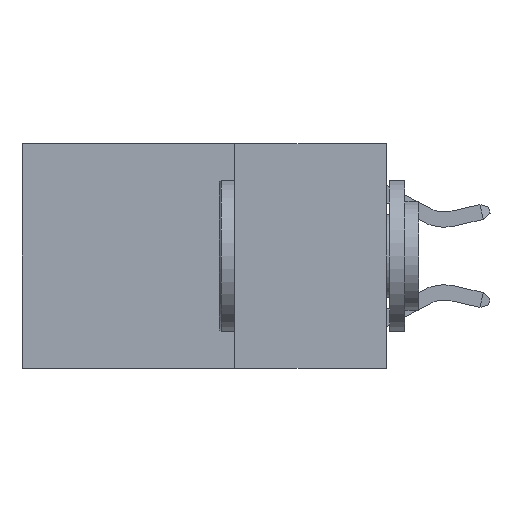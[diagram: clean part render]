
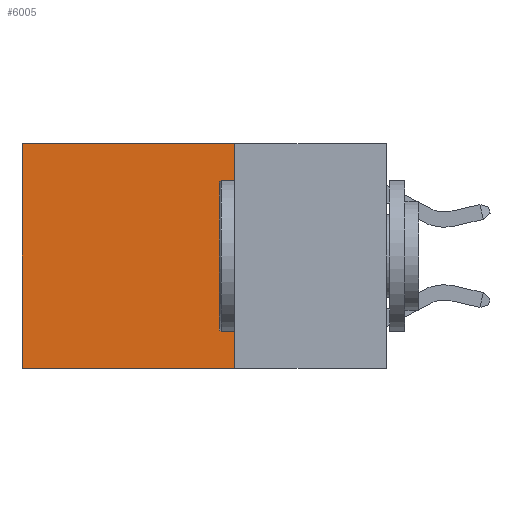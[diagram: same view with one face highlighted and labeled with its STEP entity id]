
A CAD part, left-side view. The second image highlights one B-rep face of the part: STEP entity #6005.
In plain terms, the highlighted planar face has unit normal (-1, 0, 0).
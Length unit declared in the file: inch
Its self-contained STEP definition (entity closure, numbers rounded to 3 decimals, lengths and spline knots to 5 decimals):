
#1606 = CARTESIAN_POINT ( 'NONE',  ( 0.2625, 0.25, 0. ) ) ;
#1616 = VECTOR ( 'NONE', #11368, 39.37008 ) ;
#2051 = DIRECTION ( 'NONE',  ( 0., 1., 0. ) ) ;
#2196 = CARTESIAN_POINT ( 'NONE',  ( 0.2625, 0.25, -0.37 ) ) ;
#2661 = ORIENTED_EDGE ( 'NONE', *, *, #12809, .F. ) ;
#2787 = VERTEX_POINT ( 'NONE', #15792 ) ;
#3912 = EDGE_CURVE ( 'NONE', #16897, #20954, #8694, .T. ) ;
#4120 = CARTESIAN_POINT ( 'NONE',  ( 0.2625, 0.25, -0.37 ) ) ;
#4448 = LINE ( 'NONE', #11526, #12415 ) ;
#4770 = DIRECTION ( 'NONE',  ( 0., 0., -1. ) ) ;
#5653 = ORIENTED_EDGE ( 'NONE', *, *, #3912, .F. ) ;
#6005 = ADVANCED_FACE ( 'NONE', ( #11498 ), #17484, .F. ) ;
#6724 = DIRECTION ( 'NONE',  ( 0., 1., 0. ) ) ;
#7511 = DIRECTION ( 'NONE',  ( 1., 0., 0. ) ) ;
#8415 = CARTESIAN_POINT ( 'NONE',  ( 0.2625, 0.6, -0.37 ) ) ;
#8437 = EDGE_LOOP ( 'NONE', ( #17320, #5653, #2661, #11822 ) ) ;
#8694 = LINE ( 'NONE', #2196, #13997 ) ;
#8998 = LINE ( 'NONE', #15191, #18044 ) ;
#11368 = DIRECTION ( 'NONE',  ( 0., 0., -1. ) ) ;
#11498 = FACE_OUTER_BOUND ( 'NONE', #8437, .T. ) ;
#11526 = CARTESIAN_POINT ( 'NONE',  ( 0.2625, 0.6, 0. ) ) ;
#11822 = ORIENTED_EDGE ( 'NONE', *, *, #18336, .T. ) ;
#12415 = VECTOR ( 'NONE', #4770, 39.37008 ) ;
#12809 = EDGE_CURVE ( 'NONE', #15316, #16897, #14433, .T. ) ;
#13997 = VECTOR ( 'NONE', #2051, 39.37008 ) ;
#14433 = LINE ( 'NONE', #14573, #1616 ) ;
#14573 = CARTESIAN_POINT ( 'NONE',  ( 0.2625, 0.25, 0. ) ) ;
#15191 = CARTESIAN_POINT ( 'NONE',  ( 0.2625, 0.25, 0. ) ) ;
#15316 = VERTEX_POINT ( 'NONE', #1606 ) ;
#15766 = DIRECTION ( 'NONE',  ( 0., 0., -1. ) ) ;
#15792 = CARTESIAN_POINT ( 'NONE',  ( 0.2625, 0.6, 0. ) ) ;
#16897 = VERTEX_POINT ( 'NONE', #4120 ) ;
#17320 = ORIENTED_EDGE ( 'NONE', *, *, #18469, .T. ) ;
#17484 = PLANE ( 'NONE',  #17532 ) ;
#17532 = AXIS2_PLACEMENT_3D ( 'NONE', #17705, #7511, #15766 ) ;
#17705 = CARTESIAN_POINT ( 'NONE',  ( 0.2625, 0.25, 0. ) ) ;
#18044 = VECTOR ( 'NONE', #6724, 39.37008 ) ;
#18336 = EDGE_CURVE ( 'NONE', #15316, #2787, #8998, .T. ) ;
#18469 = EDGE_CURVE ( 'NONE', #2787, #20954, #4448, .T. ) ;
#20954 = VERTEX_POINT ( 'NONE', #8415 ) ;
